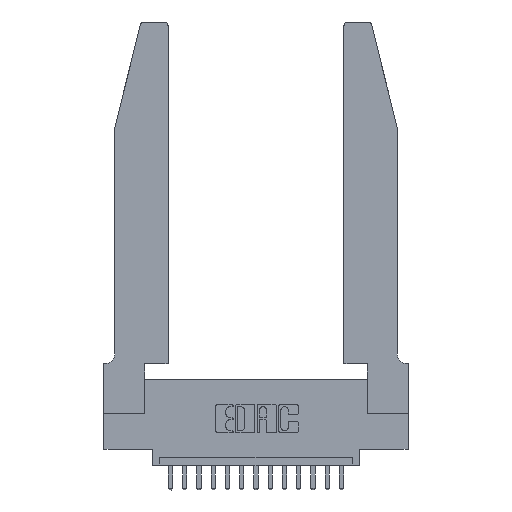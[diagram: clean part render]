
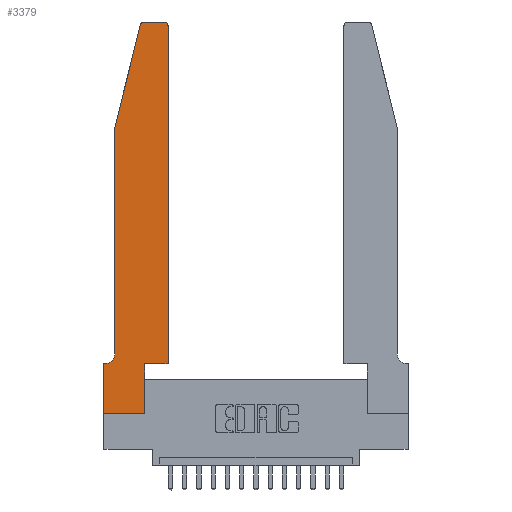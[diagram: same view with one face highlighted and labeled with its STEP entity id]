
A CAD part, top view. The second image highlights one B-rep face of the part: STEP entity #3379.
In plain terms, the highlighted planar face has unit normal (0, 0, 1).
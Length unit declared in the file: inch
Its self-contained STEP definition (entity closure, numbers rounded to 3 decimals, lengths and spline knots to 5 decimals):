
#88 = VERTEX_POINT ( 'NONE', #15623 ) ;
#321 = DIRECTION ( 'NONE',  ( 1., 0., 0. ) ) ;
#445 = EDGE_CURVE ( 'NONE', #893, #11861, #11132, .T. ) ;
#516 = CARTESIAN_POINT ( 'NONE',  ( 0.2865, 0.35, 0.37 ) ) ;
#546 = CARTESIAN_POINT ( 'NONE',  ( 0.4205, 2.72, 0.37 ) ) ;
#725 = CARTESIAN_POINT ( 'NONE',  ( 0.0055, 0.35, 0.37 ) ) ;
#844 = CARTESIAN_POINT ( 'NONE',  ( 0.0755, 0.35, 0.37 ) ) ;
#893 = VERTEX_POINT ( 'NONE', #516 ) ;
#1012 = EDGE_CURVE ( 'NONE', #2338, #4308, #15617, .T. ) ;
#1062 = ORIENTED_EDGE ( 'NONE', *, *, #2292, .T. ) ;
#1066 = DIRECTION ( 'NONE',  ( 1., 0., 0. ) ) ;
#1126 = PLANE ( 'NONE',  #14694 ) ;
#1258 = EDGE_CURVE ( 'NONE', #11861, #9137, #13801, .T. ) ;
#1817 = VECTOR ( 'NONE', #17219, 39.37008 ) ;
#1822 = EDGE_CURVE ( 'NONE', #15098, #2373, #5169, .T. ) ;
#1893 = ORIENTED_EDGE ( 'NONE', *, *, #3171, .T. ) ;
#1962 = CIRCLE ( 'NONE', #8351, 0.03 ) ;
#2292 = EDGE_CURVE ( 'NONE', #9761, #2338, #6251, .T. ) ;
#2338 = VERTEX_POINT ( 'NONE', #7351 ) ;
#2373 = VERTEX_POINT ( 'NONE', #10688 ) ;
#2811 = CARTESIAN_POINT ( 'NONE',  ( 0.2605, 2.75, 0.37 ) ) ;
#2852 = ORIENTED_EDGE ( 'NONE', *, *, #6239, .T. ) ;
#3053 = ORIENTED_EDGE ( 'NONE', *, *, #1822, .T. ) ;
#3171 = EDGE_CURVE ( 'NONE', #6197, #893, #9241, .T. ) ;
#3379 = ADVANCED_FACE ( 'NONE', ( #12844 ), #1126, .T. ) ;
#3849 = VECTOR ( 'NONE', #5115, 39.37008 ) ;
#3903 = CIRCLE ( 'NONE', #17716, 0.07 ) ;
#4011 = DIRECTION ( 'NONE',  ( 0., -1., 0. ) ) ;
#4170 = CARTESIAN_POINT ( 'NONE',  ( 0.4505, 0.35, 0.37 ) ) ;
#4308 = VERTEX_POINT ( 'NONE', #6426 ) ;
#4423 = CARTESIAN_POINT ( 'NONE',  ( 0.284, 2.72, 0.37 ) ) ;
#4587 = CARTESIAN_POINT ( 'NONE',  ( 0.284, 2.75, 0.37 ) ) ;
#5052 = EDGE_CURVE ( 'NONE', #4308, #15098, #3903, .T. ) ;
#5115 = DIRECTION ( 'NONE',  ( 0., -1., 0. ) ) ;
#5169 = LINE ( 'NONE', #844, #8327 ) ;
#5315 = ORIENTED_EDGE ( 'NONE', *, *, #1258, .T. ) ;
#5324 = VECTOR ( 'NONE', #8430, 39.37008 ) ;
#5329 = CARTESIAN_POINT ( 'NONE',  ( 0.0755, 2., 0.37 ) ) ;
#5508 = DIRECTION ( 'NONE',  ( 0., 0., -1. ) ) ;
#5522 = EDGE_LOOP ( 'NONE', ( #8567, #6442, #1062, #9992, #9949, #3053, #2852, #11645, #1893, #14777, #5315, #15624 ) ) ;
#5830 = DIRECTION ( 'NONE',  ( 0., 0., 1. ) ) ;
#6197 = VERTEX_POINT ( 'NONE', #17625 ) ;
#6239 = EDGE_CURVE ( 'NONE', #2373, #88, #15383, .T. ) ;
#6248 = LINE ( 'NONE', #18721, #15999 ) ;
#6251 = LINE ( 'NONE', #5329, #11512 ) ;
#6397 = CIRCLE ( 'NONE', #18286, 0.03 ) ;
#6426 = CARTESIAN_POINT ( 'NONE',  ( 0.0755, 0.42, 0.37 ) ) ;
#6442 = ORIENTED_EDGE ( 'NONE', *, *, #13273, .T. ) ;
#7139 = CARTESIAN_POINT ( 'NONE',  ( 0.4205, 2.75, 0.37 ) ) ;
#7351 = CARTESIAN_POINT ( 'NONE',  ( 0.0755, 2., 0.37 ) ) ;
#8188 = DIRECTION ( 'NONE',  ( 0., 1., 0. ) ) ;
#8228 = CARTESIAN_POINT ( 'NONE',  ( 0.0755, 2., 0.37 ) ) ;
#8327 = VECTOR ( 'NONE', #15366, 39.37008 ) ;
#8351 = AXIS2_PLACEMENT_3D ( 'NONE', #546, #12119, #14025 ) ;
#8430 = DIRECTION ( 'NONE',  ( -1., 0., 0. ) ) ;
#8567 = ORIENTED_EDGE ( 'NONE', *, *, #8582, .T. ) ;
#8582 = EDGE_CURVE ( 'NONE', #11882, #10163, #17994, .T. ) ;
#8588 = DIRECTION ( 'NONE',  ( 1., 0., 0. ) ) ;
#9137 = VERTEX_POINT ( 'NONE', #9650 ) ;
#9241 = LINE ( 'NONE', #13838, #16889 ) ;
#9292 = CARTESIAN_POINT ( 'NONE',  ( 0.4505, 0.35, 0.37 ) ) ;
#9307 = EDGE_CURVE ( 'NONE', #9137, #11882, #1962, .T. ) ;
#9650 = CARTESIAN_POINT ( 'NONE',  ( 0.4505, 2.72, 0.37 ) ) ;
#9761 = VERTEX_POINT ( 'NONE', #12131 ) ;
#9949 = ORIENTED_EDGE ( 'NONE', *, *, #5052, .T. ) ;
#9992 = ORIENTED_EDGE ( 'NONE', *, *, #1012, .T. ) ;
#10107 = CARTESIAN_POINT ( 'NONE',  ( 0.4505, 0.35, 0.37 ) ) ;
#10163 = VERTEX_POINT ( 'NONE', #4587 ) ;
#10688 = CARTESIAN_POINT ( 'NONE',  ( 0., 0.35, 0.37 ) ) ;
#11132 = LINE ( 'NONE', #9292, #13144 ) ;
#11263 = CARTESIAN_POINT ( 'NONE',  ( 0., 0.35, 0.37 ) ) ;
#11285 = EDGE_CURVE ( 'NONE', #88, #6197, #6248, .T. ) ;
#11512 = VECTOR ( 'NONE', #16895, 39.37008 ) ;
#11645 = ORIENTED_EDGE ( 'NONE', *, *, #11285, .T. ) ;
#11791 = VECTOR ( 'NONE', #4011, 39.37008 ) ;
#11861 = VERTEX_POINT ( 'NONE', #10107 ) ;
#11882 = VERTEX_POINT ( 'NONE', #7139 ) ;
#12119 = DIRECTION ( 'NONE',  ( 0., 0., 1. ) ) ;
#12131 = CARTESIAN_POINT ( 'NONE',  ( 0.25487, 2.72718, 0.37 ) ) ;
#12823 = DIRECTION ( 'NONE',  ( 0., 0., 1. ) ) ;
#12844 = FACE_OUTER_BOUND ( 'NONE', #5522, .T. ) ;
#13144 = VECTOR ( 'NONE', #16360, 39.37008 ) ;
#13273 = EDGE_CURVE ( 'NONE', #10163, #9761, #6397, .T. ) ;
#13801 = LINE ( 'NONE', #4170, #1817 ) ;
#13838 = CARTESIAN_POINT ( 'NONE',  ( 0.2865, 0.35, 0.37 ) ) ;
#13905 = CARTESIAN_POINT ( 'NONE',  ( 0., 0., 0.37 ) ) ;
#14025 = DIRECTION ( 'NONE',  ( 1., 0., 0. ) ) ;
#14694 = AXIS2_PLACEMENT_3D ( 'NONE', #11263, #12823, #1066 ) ;
#14777 = ORIENTED_EDGE ( 'NONE', *, *, #445, .T. ) ;
#15098 = VERTEX_POINT ( 'NONE', #725 ) ;
#15366 = DIRECTION ( 'NONE',  ( -1., 0., 0. ) ) ;
#15383 = LINE ( 'NONE', #13905, #3849 ) ;
#15470 = CARTESIAN_POINT ( 'NONE',  ( 0.0055, 0.42, 0.37 ) ) ;
#15617 = LINE ( 'NONE', #8228, #11791 ) ;
#15623 = CARTESIAN_POINT ( 'NONE',  ( 0., 0., 0.37 ) ) ;
#15624 = ORIENTED_EDGE ( 'NONE', *, *, #9307, .T. ) ;
#15999 = VECTOR ( 'NONE', #8588, 39.37008 ) ;
#16360 = DIRECTION ( 'NONE',  ( 1., 0., 0. ) ) ;
#16889 = VECTOR ( 'NONE', #8188, 39.37008 ) ;
#16895 = DIRECTION ( 'NONE',  ( -0.239, -0.971, 0. ) ) ;
#17219 = DIRECTION ( 'NONE',  ( 0., 1., 0. ) ) ;
#17625 = CARTESIAN_POINT ( 'NONE',  ( 0.2865, 0., 0.37 ) ) ;
#17716 = AXIS2_PLACEMENT_3D ( 'NONE', #15470, #5508, #18472 ) ;
#17994 = LINE ( 'NONE', #2811, #5324 ) ;
#18286 = AXIS2_PLACEMENT_3D ( 'NONE', #4423, #5830, #321 ) ;
#18472 = DIRECTION ( 'NONE',  ( -1., 0., 0. ) ) ;
#18721 = CARTESIAN_POINT ( 'NONE',  ( 0., 0., 0.37 ) ) ;
